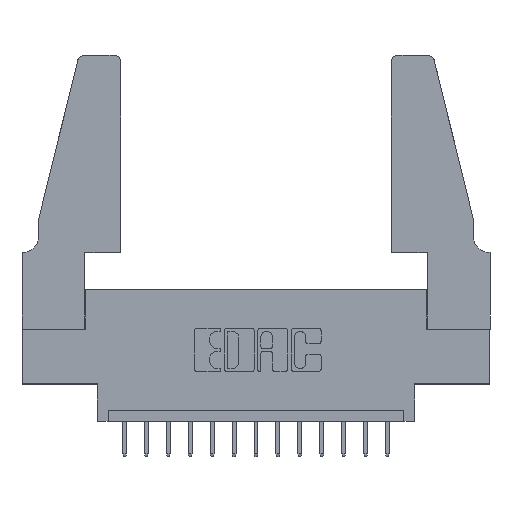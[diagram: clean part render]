
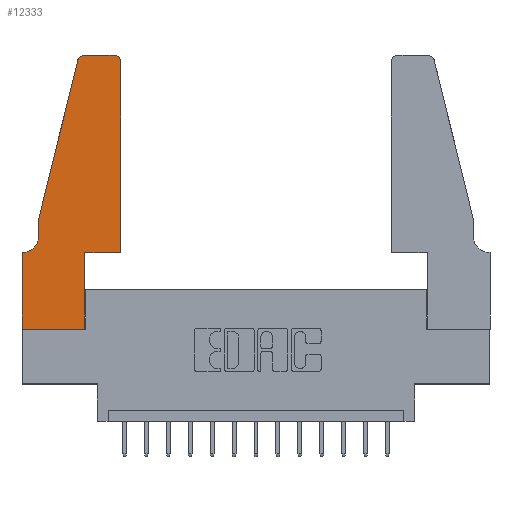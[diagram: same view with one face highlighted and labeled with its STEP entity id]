
A CAD part, top view. The second image highlights one B-rep face of the part: STEP entity #12333.
In plain terms, the highlighted planar face has unit normal (0, 0, 1).
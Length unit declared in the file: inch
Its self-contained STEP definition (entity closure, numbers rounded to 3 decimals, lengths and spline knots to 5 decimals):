
#140 = DIRECTION ( 'NONE',  ( 1., 0., 0. ) ) ;
#245 = CARTESIAN_POINT ( 'NONE',  ( 0.2865, 0.35, 0.37 ) ) ;
#569 = VERTEX_POINT ( 'NONE', #14291 ) ;
#607 = ORIENTED_EDGE ( 'NONE', *, *, #7506, .T. ) ;
#813 = EDGE_CURVE ( 'NONE', #5039, #13173, #15440, .T. ) ;
#1014 = ORIENTED_EDGE ( 'NONE', *, *, #14256, .T. ) ;
#1246 = CARTESIAN_POINT ( 'NONE',  ( 0., 0., 0.37 ) ) ;
#1613 = DIRECTION ( 'NONE',  ( 0., 0., 1. ) ) ;
#2070 = EDGE_CURVE ( 'NONE', #11960, #2157, #4344, .T. ) ;
#2142 = VECTOR ( 'NONE', #2690, 39.37008 ) ;
#2143 = CARTESIAN_POINT ( 'NONE',  ( 0.0755, 0.5, 0.37 ) ) ;
#2157 = VERTEX_POINT ( 'NONE', #7262 ) ;
#2159 = CARTESIAN_POINT ( 'NONE',  ( 0.4505, 0.35, 0.37 ) ) ;
#2453 = CIRCLE ( 'NONE', #14368, 0.03 ) ;
#2589 = DIRECTION ( 'NONE',  ( 0., 0., 1. ) ) ;
#2660 = VECTOR ( 'NONE', #10245, 39.37008 ) ;
#2690 = DIRECTION ( 'NONE',  ( 0., 1., 0. ) ) ;
#2764 = CARTESIAN_POINT ( 'NONE',  ( 0.0755, 0.35, 0.37 ) ) ;
#3028 = CARTESIAN_POINT ( 'NONE',  ( 0.25487, 1.22718, 0.37 ) ) ;
#3357 = VECTOR ( 'NONE', #140, 39.37008 ) ;
#3468 = ORIENTED_EDGE ( 'NONE', *, *, #10663, .T. ) ;
#3625 = CARTESIAN_POINT ( 'NONE',  ( 0.284, 1.25, 0.37 ) ) ;
#4344 = LINE ( 'NONE', #15245, #12641 ) ;
#4358 = DIRECTION ( 'NONE',  ( -1., 0., 0. ) ) ;
#4877 = CARTESIAN_POINT ( 'NONE',  ( 0.4505, 1.22, 0.37 ) ) ;
#5037 = EDGE_CURVE ( 'NONE', #10070, #5833, #6140, .T. ) ;
#5039 = VERTEX_POINT ( 'NONE', #14164 ) ;
#5253 = CARTESIAN_POINT ( 'NONE',  ( 0., 0.35, 0.37 ) ) ;
#5378 = DIRECTION ( 'NONE',  ( -0.239, -0.971, 0. ) ) ;
#5833 = VERTEX_POINT ( 'NONE', #3625 ) ;
#6021 = CARTESIAN_POINT ( 'NONE',  ( 0.284, 1.22, 0.37 ) ) ;
#6088 = ORIENTED_EDGE ( 'NONE', *, *, #2070, .T. ) ;
#6140 = LINE ( 'NONE', #13006, #15290 ) ;
#6152 = VECTOR ( 'NONE', #5378, 39.37008 ) ;
#6432 = CARTESIAN_POINT ( 'NONE',  ( 0.0755, 0.5, 0.37 ) ) ;
#6519 = VECTOR ( 'NONE', #10818, 39.37008 ) ;
#6667 = AXIS2_PLACEMENT_3D ( 'NONE', #6021, #2589, #11207 ) ;
#6842 = EDGE_CURVE ( 'NONE', #569, #7687, #8770, .T. ) ;
#7119 = LINE ( 'NONE', #6432, #6152 ) ;
#7262 = CARTESIAN_POINT ( 'NONE',  ( 0.0755, 0.42, 0.37 ) ) ;
#7506 = EDGE_CURVE ( 'NONE', #13173, #15456, #7579, .T. ) ;
#7579 = LINE ( 'NONE', #14550, #3357 ) ;
#7614 = PLANE ( 'NONE',  #14268 ) ;
#7629 = VERTEX_POINT ( 'NONE', #8423 ) ;
#7687 = VERTEX_POINT ( 'NONE', #4877 ) ;
#7900 = LINE ( 'NONE', #245, #2142 ) ;
#8046 = EDGE_LOOP ( 'NONE', ( #14959, #10231, #13956, #6088, #1014, #3468, #14414, #607, #13869, #11842, #13084, #11440 ) ) ;
#8423 = CARTESIAN_POINT ( 'NONE',  ( 0.0055, 0.35, 0.37 ) ) ;
#8770 = LINE ( 'NONE', #14271, #15959 ) ;
#8812 = VECTOR ( 'NONE', #11107, 39.37008 ) ;
#9034 = DIRECTION ( 'NONE',  ( 0., -1., 0. ) ) ;
#9216 = LINE ( 'NONE', #2764, #2660 ) ;
#9279 = DIRECTION ( 'NONE',  ( 0., 1., 0. ) ) ;
#9439 = EDGE_CURVE ( 'NONE', #15456, #12931, #7900, .T. ) ;
#9810 = CARTESIAN_POINT ( 'NONE',  ( 0.2865, 0., 0.37 ) ) ;
#10070 = VERTEX_POINT ( 'NONE', #11242 ) ;
#10231 = ORIENTED_EDGE ( 'NONE', *, *, #14203, .T. ) ;
#10245 = DIRECTION ( 'NONE',  ( -1., 0., 0. ) ) ;
#10332 = CARTESIAN_POINT ( 'NONE',  ( 0.2865, 0.35, 0.37 ) ) ;
#10663 = EDGE_CURVE ( 'NONE', #7629, #5039, #9216, .T. ) ;
#10722 = EDGE_CURVE ( 'NONE', #12931, #569, #13121, .T. ) ;
#10781 = DIRECTION ( 'NONE',  ( 0., 0., 1. ) ) ;
#10818 = DIRECTION ( 'NONE',  ( 1., 0., 0. ) ) ;
#10830 = VERTEX_POINT ( 'NONE', #3028 ) ;
#10997 = CARTESIAN_POINT ( 'NONE',  ( 0.4205, 1.22, 0.37 ) ) ;
#11107 = DIRECTION ( 'NONE',  ( 0., -1., 0. ) ) ;
#11207 = DIRECTION ( 'NONE',  ( 1., 0., 0. ) ) ;
#11242 = CARTESIAN_POINT ( 'NONE',  ( 0.4205, 1.25, 0.37 ) ) ;
#11307 = EDGE_CURVE ( 'NONE', #7687, #10070, #2453, .T. ) ;
#11440 = ORIENTED_EDGE ( 'NONE', *, *, #11307, .T. ) ;
#11457 = FACE_OUTER_BOUND ( 'NONE', #8046, .T. ) ;
#11482 = DIRECTION ( 'NONE',  ( 1., 0., 0. ) ) ;
#11842 = ORIENTED_EDGE ( 'NONE', *, *, #10722, .T. ) ;
#11960 = VERTEX_POINT ( 'NONE', #2143 ) ;
#12333 = ADVANCED_FACE ( 'NONE', ( #11457 ), #7614, .T. ) ;
#12641 = VECTOR ( 'NONE', #9034, 39.37008 ) ;
#12931 = VERTEX_POINT ( 'NONE', #10332 ) ;
#13006 = CARTESIAN_POINT ( 'NONE',  ( 0.2605, 1.25, 0.37 ) ) ;
#13084 = ORIENTED_EDGE ( 'NONE', *, *, #6842, .T. ) ;
#13121 = LINE ( 'NONE', #2159, #6519 ) ;
#13173 = VERTEX_POINT ( 'NONE', #15284 ) ;
#13203 = CARTESIAN_POINT ( 'NONE',  ( 0.0055, 0.42, 0.37 ) ) ;
#13220 = DIRECTION ( 'NONE',  ( -1., 0., 0. ) ) ;
#13282 = DIRECTION ( 'NONE',  ( 1., 0., 0. ) ) ;
#13869 = ORIENTED_EDGE ( 'NONE', *, *, #9439, .T. ) ;
#13956 = ORIENTED_EDGE ( 'NONE', *, *, #15766, .T. ) ;
#14164 = CARTESIAN_POINT ( 'NONE',  ( 0., 0.35, 0.37 ) ) ;
#14175 = AXIS2_PLACEMENT_3D ( 'NONE', #13203, #14475, #4358 ) ;
#14203 = EDGE_CURVE ( 'NONE', #5833, #10830, #14780, .T. ) ;
#14256 = EDGE_CURVE ( 'NONE', #2157, #7629, #15564, .T. ) ;
#14268 = AXIS2_PLACEMENT_3D ( 'NONE', #5253, #1613, #11482 ) ;
#14271 = CARTESIAN_POINT ( 'NONE',  ( 0.4505, 0.35, 0.37 ) ) ;
#14291 = CARTESIAN_POINT ( 'NONE',  ( 0.4505, 0.35, 0.37 ) ) ;
#14368 = AXIS2_PLACEMENT_3D ( 'NONE', #10997, #10781, #13282 ) ;
#14414 = ORIENTED_EDGE ( 'NONE', *, *, #813, .T. ) ;
#14475 = DIRECTION ( 'NONE',  ( 0., 0., -1. ) ) ;
#14550 = CARTESIAN_POINT ( 'NONE',  ( 0., 0., 0.37 ) ) ;
#14780 = CIRCLE ( 'NONE', #6667, 0.03 ) ;
#14959 = ORIENTED_EDGE ( 'NONE', *, *, #5037, .T. ) ;
#15245 = CARTESIAN_POINT ( 'NONE',  ( 0.0755, 0.5, 0.37 ) ) ;
#15284 = CARTESIAN_POINT ( 'NONE',  ( 0., 0., 0.37 ) ) ;
#15290 = VECTOR ( 'NONE', #13220, 39.37008 ) ;
#15440 = LINE ( 'NONE', #1246, #8812 ) ;
#15456 = VERTEX_POINT ( 'NONE', #9810 ) ;
#15564 = CIRCLE ( 'NONE', #14175, 0.07 ) ;
#15766 = EDGE_CURVE ( 'NONE', #10830, #11960, #7119, .T. ) ;
#15959 = VECTOR ( 'NONE', #9279, 39.37008 ) ;
